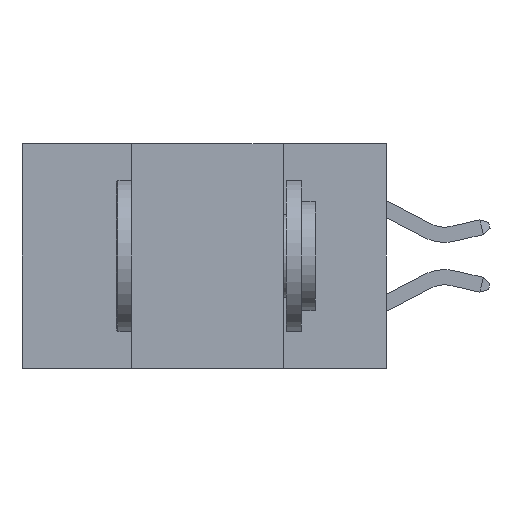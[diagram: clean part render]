
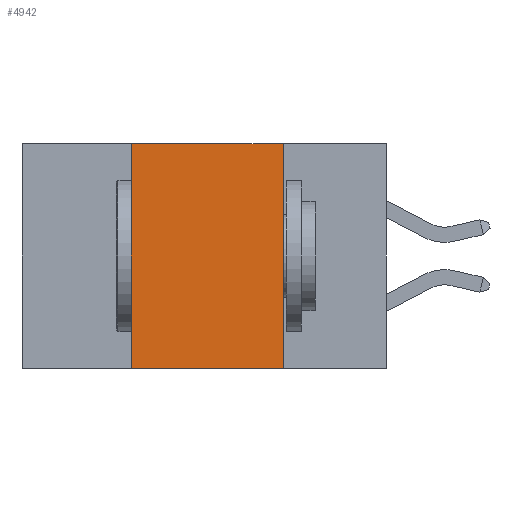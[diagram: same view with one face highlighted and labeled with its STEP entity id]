
A CAD part, left-side view. The second image highlights one B-rep face of the part: STEP entity #4942.
In plain terms, the highlighted planar face has unit normal (-1, 0, 0).
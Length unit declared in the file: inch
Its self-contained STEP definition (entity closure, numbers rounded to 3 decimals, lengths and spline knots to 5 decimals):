
#184 = EDGE_CURVE ( 'NONE', #10138, #2910, #3353, .T. ) ;
#540 = ORIENTED_EDGE ( 'NONE', *, *, #6600, .T. ) ;
#1453 = LINE ( 'NONE', #1662, #12034 ) ;
#1662 = CARTESIAN_POINT ( 'NONE',  ( 0., 0.6, 0. ) ) ;
#1730 = EDGE_CURVE ( 'NONE', #9661, #11913, #6697, .T. ) ;
#2033 = CARTESIAN_POINT ( 'NONE',  ( 0., 0.17, -0.37 ) ) ;
#2481 = PLANE ( 'NONE',  #5730 ) ;
#2509 = VECTOR ( 'NONE', #10000, 39.37008 ) ;
#2910 = VERTEX_POINT ( 'NONE', #13907 ) ;
#3332 = CARTESIAN_POINT ( 'NONE',  ( 0., 0.6, -0.37 ) ) ;
#3353 = LINE ( 'NONE', #7796, #9579 ) ;
#4942 = ADVANCED_FACE ( 'NONE', ( #13394 ), #2481, .F. ) ;
#5696 = ORIENTED_EDGE ( 'NONE', *, *, #184, .F. ) ;
#5730 = AXIS2_PLACEMENT_3D ( 'NONE', #13114, #6852, #6569 ) ;
#5757 = CARTESIAN_POINT ( 'NONE',  ( 0., 0.17, -0.37 ) ) ;
#6569 = DIRECTION ( 'NONE',  ( 0., 0., -1. ) ) ;
#6600 = EDGE_CURVE ( 'NONE', #10138, #11913, #9993, .T. ) ;
#6697 = LINE ( 'NONE', #5757, #2509 ) ;
#6852 = DIRECTION ( 'NONE',  ( 1., 0., 0. ) ) ;
#6858 = DIRECTION ( 'NONE',  ( 0., 0., 1. ) ) ;
#7362 = CARTESIAN_POINT ( 'NONE',  ( 0., 0.42, -0.37 ) ) ;
#7796 = CARTESIAN_POINT ( 'NONE',  ( 0., 0.42, -0.37 ) ) ;
#8043 = DIRECTION ( 'NONE',  ( 0., -1., 0. ) ) ;
#8288 = EDGE_CURVE ( 'NONE', #2910, #9661, #1453, .T. ) ;
#8784 = DIRECTION ( 'NONE',  ( 0., -1., 0. ) ) ;
#9202 = EDGE_LOOP ( 'NONE', ( #14013, #12837, #5696, #540 ) ) ;
#9579 = VECTOR ( 'NONE', #6858, 39.37008 ) ;
#9661 = VERTEX_POINT ( 'NONE', #13643 ) ;
#9993 = LINE ( 'NONE', #3332, #12190 ) ;
#10000 = DIRECTION ( 'NONE',  ( 0., 0., -1. ) ) ;
#10138 = VERTEX_POINT ( 'NONE', #7362 ) ;
#11913 = VERTEX_POINT ( 'NONE', #2033 ) ;
#12034 = VECTOR ( 'NONE', #8043, 39.37008 ) ;
#12190 = VECTOR ( 'NONE', #8784, 39.37008 ) ;
#12837 = ORIENTED_EDGE ( 'NONE', *, *, #8288, .F. ) ;
#13114 = CARTESIAN_POINT ( 'NONE',  ( 0., 0.6, 0. ) ) ;
#13394 = FACE_OUTER_BOUND ( 'NONE', #9202, .T. ) ;
#13643 = CARTESIAN_POINT ( 'NONE',  ( 0., 0.17, 0. ) ) ;
#13907 = CARTESIAN_POINT ( 'NONE',  ( 0., 0.42, 0. ) ) ;
#14013 = ORIENTED_EDGE ( 'NONE', *, *, #1730, .F. ) ;
